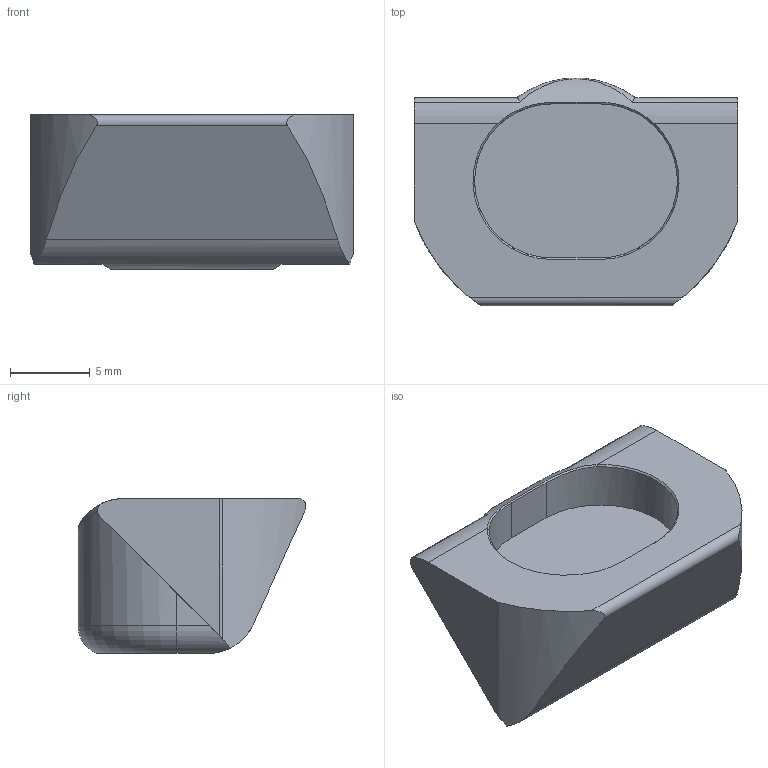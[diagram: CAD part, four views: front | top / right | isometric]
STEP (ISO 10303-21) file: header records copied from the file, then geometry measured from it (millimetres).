
FILE_DESCRIPTION(/* description */ (''),/* implementation_level */ '2;1');
FILE_NAME(/* name */ 'Tube Anti-Rotation Plug.stp',/* time_stamp */ '2020-09-06T15:27:48-05:00',/* author */ ('johne'),/* organization */ (''),/* preprocessor_version */ 'ST-DEVELOPER v18',/* originating_system */ 'Autodesk Inventor 2020',/* authorisation */ '');
FILE_SCHEMA (('AUTOMOTIVE_DESIGN { 1 0 10303 214 3 1 1 }'));
Length unit declared in the file: inch
Products named in the file (1): rotation stop
Bounding box: 20.32 x 14.33 x 9.74 mm (x, y, z)
Volume: 1487.3 mm3; surface area: 1039.3 mm2
Topology: 1 solids, 1 shells, 38 faces, 100 edges, 64 vertices
Faces by surface type: cylinder 16, plane 14, bspline 5, cone 2, torus 1
Entity records: 1438 total; most frequent: CARTESIAN_POINT 493, ORIENTED_EDGE 200, DIRECTION 172, EDGE_CURVE 100, VERTEX_POINT 64, AXIS2_PLACEMENT_3D 62, LINE 48, VECTOR 48
